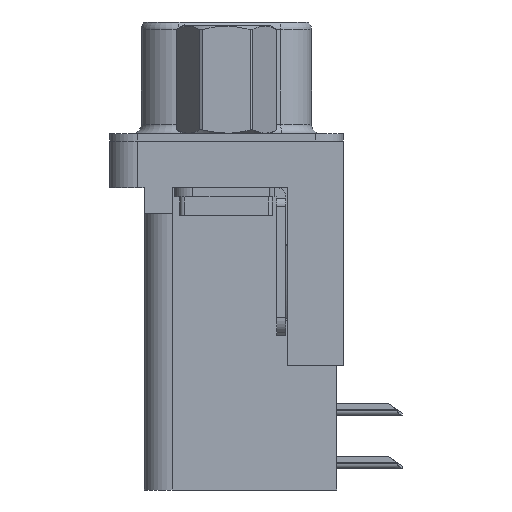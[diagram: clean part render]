
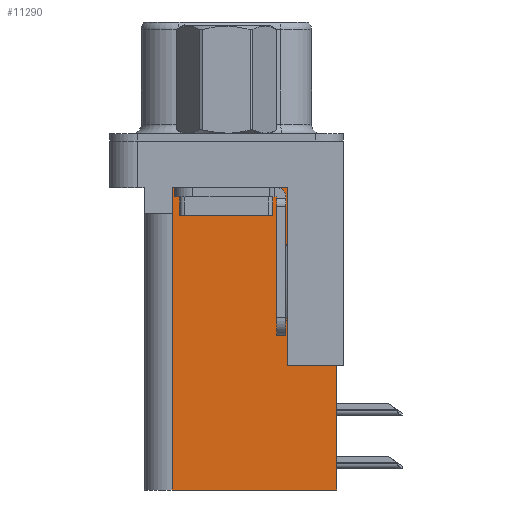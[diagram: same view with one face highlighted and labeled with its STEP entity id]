
A CAD part, left-side view. The second image highlights one B-rep face of the part: STEP entity #11290.
In plain terms, the highlighted planar face has unit normal (-1, 0, 0).
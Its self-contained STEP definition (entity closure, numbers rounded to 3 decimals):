
#361 = CARTESIAN_POINT ( 'NONE',  ( 3.79, 0., -3.9 ) ) ;
#427 = VECTOR ( 'NONE', #786, 1000. ) ;
#516 = CARTESIAN_POINT ( 'NONE',  ( 3.79, -3.295, -2.5 ) ) ;
#786 = DIRECTION ( 'NONE',  ( 0., 0., 1. ) ) ;
#858 = ORIENTED_EDGE ( 'NONE', *, *, #30576, .T. ) ;
#933 = VERTEX_POINT ( 'NONE', #19812 ) ;
#1487 = LINE ( 'NONE', #25250, #15494 ) ;
#1758 = VERTEX_POINT ( 'NONE', #24937 ) ;
#2171 = DIRECTION ( 'NONE',  ( 0., 1., 0. ) ) ;
#2272 = EDGE_CURVE ( 'NONE', #12713, #933, #28261, .T. ) ;
#2999 = CARTESIAN_POINT ( 'NONE',  ( 3.79, 2.895, -2.5 ) ) ;
#3049 = CARTESIAN_POINT ( 'NONE',  ( 3.79, 2.895, -3.9 ) ) ;
#3350 = LINE ( 'NONE', #22350, #16445 ) ;
#3638 = ORIENTED_EDGE ( 'NONE', *, *, #2272, .F. ) ;
#3713 = EDGE_LOOP ( 'NONE', ( #15651, #15253, #22340, #19925, #11096, #3638, #11960, #858 ) ) ;
#3746 = DIRECTION ( 'NONE',  ( 0., 1., 0. ) ) ;
#4550 = VECTOR ( 'NONE', #24169, 1000. ) ;
#5863 = LINE ( 'NONE', #516, #18912 ) ;
#6458 = VERTEX_POINT ( 'NONE', #16715 ) ;
#7776 = LINE ( 'NONE', #361, #21677 ) ;
#8180 = CARTESIAN_POINT ( 'NONE',  ( 3.79, -5.925, -12.05 ) ) ;
#8436 = VERTEX_POINT ( 'NONE', #10600 ) ;
#8570 = EDGE_CURVE ( 'NONE', #8436, #14775, #5863, .T. ) ;
#9126 = EDGE_CURVE ( 'NONE', #23469, #1758, #7776, .T. ) ;
#9522 = DIRECTION ( 'NONE',  ( 0., 1., 0. ) ) ;
#10600 = CARTESIAN_POINT ( 'NONE',  ( 3.79, -3.295, -2.5 ) ) ;
#10870 = FACE_OUTER_BOUND ( 'NONE', #3713, .T. ) ;
#11096 = ORIENTED_EDGE ( 'NONE', *, *, #16966, .F. ) ;
#11290 = ADVANCED_FACE ( 'NONE', ( #10870 ), #16750, .F. ) ;
#11352 = CARTESIAN_POINT ( 'NONE',  ( 3.79, 2.925, -18.76 ) ) ;
#11491 = LINE ( 'NONE', #3049, #4550 ) ;
#11960 = ORIENTED_EDGE ( 'NONE', *, *, #18561, .T. ) ;
#12713 = VERTEX_POINT ( 'NONE', #8180 ) ;
#14463 = AXIS2_PLACEMENT_3D ( 'NONE', #32234, #19389, #3746 ) ;
#14775 = VERTEX_POINT ( 'NONE', #2999 ) ;
#15135 = CARTESIAN_POINT ( 'NONE',  ( 3.79, -5.925, -2. ) ) ;
#15253 = ORIENTED_EDGE ( 'NONE', *, *, #32633, .T. ) ;
#15324 = DIRECTION ( 'NONE',  ( 0., 0., -1. ) ) ;
#15494 = VECTOR ( 'NONE', #9522, 1000. ) ;
#15651 = ORIENTED_EDGE ( 'NONE', *, *, #8570, .T. ) ;
#16150 = DIRECTION ( 'NONE',  ( 0., 1., 0. ) ) ;
#16445 = VECTOR ( 'NONE', #24996, 1000. ) ;
#16715 = CARTESIAN_POINT ( 'NONE',  ( 3.79, -3.295, -12.05 ) ) ;
#16750 = PLANE ( 'NONE',  #14463 ) ;
#16966 = EDGE_CURVE ( 'NONE', #933, #31529, #1487, .T. ) ;
#17853 = LINE ( 'NONE', #20510, #24870 ) ;
#18561 = EDGE_CURVE ( 'NONE', #12713, #6458, #17853, .T. ) ;
#18912 = VECTOR ( 'NONE', #18943, 1000. ) ;
#18943 = DIRECTION ( 'NONE',  ( 0., 1., 0. ) ) ;
#19389 = DIRECTION ( 'NONE',  ( 1., 0., 0. ) ) ;
#19812 = CARTESIAN_POINT ( 'NONE',  ( 3.79, -5.925, -18.76 ) ) ;
#19925 = ORIENTED_EDGE ( 'NONE', *, *, #22825, .F. ) ;
#20510 = CARTESIAN_POINT ( 'NONE',  ( 3.79, -6.295, -12.05 ) ) ;
#21273 = VECTOR ( 'NONE', #15324, 1000. ) ;
#21449 = LINE ( 'NONE', #29695, #427 ) ;
#21677 = VECTOR ( 'NONE', #16150, 1000. ) ;
#22340 = ORIENTED_EDGE ( 'NONE', *, *, #9126, .T. ) ;
#22350 = CARTESIAN_POINT ( 'NONE',  ( 3.79, 2.925, -18.76 ) ) ;
#22825 = EDGE_CURVE ( 'NONE', #31529, #1758, #3350, .T. ) ;
#23469 = VERTEX_POINT ( 'NONE', #33353 ) ;
#24169 = DIRECTION ( 'NONE',  ( 0., 0., -1. ) ) ;
#24870 = VECTOR ( 'NONE', #2171, 1000. ) ;
#24937 = CARTESIAN_POINT ( 'NONE',  ( 3.79, 2.925, -3.9 ) ) ;
#24996 = DIRECTION ( 'NONE',  ( 0., 0., 1. ) ) ;
#25250 = CARTESIAN_POINT ( 'NONE',  ( 3.79, -3.295, -18.76 ) ) ;
#28261 = LINE ( 'NONE', #15135, #21273 ) ;
#29695 = CARTESIAN_POINT ( 'NONE',  ( 3.79, -3.295, -18.76 ) ) ;
#30576 = EDGE_CURVE ( 'NONE', #6458, #8436, #21449, .T. ) ;
#31529 = VERTEX_POINT ( 'NONE', #11352 ) ;
#32234 = CARTESIAN_POINT ( 'NONE',  ( 3.79, -3.295, -18.76 ) ) ;
#32633 = EDGE_CURVE ( 'NONE', #14775, #23469, #11491, .T. ) ;
#33353 = CARTESIAN_POINT ( 'NONE',  ( 3.79, 2.895, -3.9 ) ) ;
